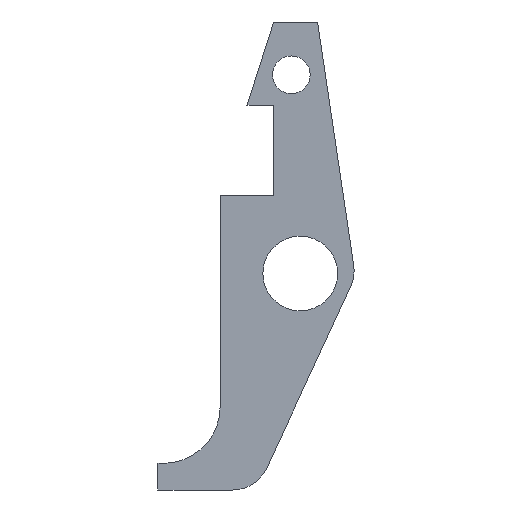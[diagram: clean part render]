
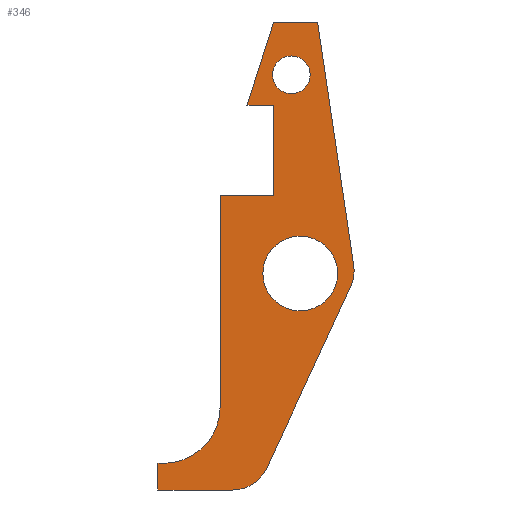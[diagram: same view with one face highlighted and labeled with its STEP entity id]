
A CAD part, front view. The second image highlights one B-rep face of the part: STEP entity #346.
In plain terms, the highlighted planar face has unit normal (0, -1, 0).
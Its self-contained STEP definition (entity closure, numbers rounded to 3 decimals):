
#17=FACE_BOUND('',#62,.T.);
#18=FACE_BOUND('',#63,.T.);
#19=CIRCLE('',#374,1.588);
#25=CIRCLE('',#383,3.175);
#26=CIRCLE('',#386,4.763);
#27=CIRCLE('',#387,3.175);
#28=CIRCLE('',#388,3.15);
#41=FACE_OUTER_BOUND('',#61,.T.);
#61=EDGE_LOOP('',(#270,#271,#272,#273,#274,#275,#276,#277,#278,#279,#280,
#281,#282,#283));
#62=EDGE_LOOP('',(#284));
#63=EDGE_LOOP('',(#285));
#76=LINE('',#503,#114);
#80=LINE('',#510,#118);
#82=LINE('',#519,#120);
#94=LINE('',#553,#132);
#96=LINE('',#557,#134);
#97=LINE('',#559,#135);
#98=LINE('',#561,#136);
#99=LINE('',#563,#137);
#100=LINE('',#567,#138);
#101=LINE('',#569,#139);
#102=LINE('',#571,#140);
#114=VECTOR('',#405,10.);
#118=VECTOR('',#411,10.);
#120=VECTOR('',#421,10.);
#132=VECTOR('',#449,10.);
#134=VECTOR('',#453,10.);
#135=VECTOR('',#454,10.);
#136=VECTOR('',#455,10.);
#137=VECTOR('',#456,10.);
#138=VECTOR('',#459,10.);
#139=VECTOR('',#460,10.);
#140=VECTOR('',#461,10.);
#152=VERTEX_POINT('',#500);
#153=VERTEX_POINT('',#502);
#155=VERTEX_POINT('',#508);
#156=VERTEX_POINT('',#512);
#158=VERTEX_POINT('',#518);
#171=VERTEX_POINT('',#548);
#172=VERTEX_POINT('',#552);
#173=VERTEX_POINT('',#556);
#174=VERTEX_POINT('',#558);
#175=VERTEX_POINT('',#560);
#176=VERTEX_POINT('',#562);
#177=VERTEX_POINT('',#564);
#178=VERTEX_POINT('',#566);
#179=VERTEX_POINT('',#568);
#180=VERTEX_POINT('',#570);
#181=VERTEX_POINT('',#573);
#184=EDGE_CURVE('',#153,#152,#76,.T.);
#188=EDGE_CURVE('',#152,#155,#80,.T.);
#189=EDGE_CURVE('',#156,#156,#19,.T.);
#192=EDGE_CURVE('',#158,#153,#82,.T.);
#207=EDGE_CURVE('',#158,#171,#25,.T.);
#209=EDGE_CURVE('',#172,#171,#94,.T.);
#211=EDGE_CURVE('',#155,#173,#96,.T.);
#212=EDGE_CURVE('',#173,#174,#97,.T.);
#213=EDGE_CURVE('',#174,#175,#98,.T.);
#214=EDGE_CURVE('',#175,#176,#99,.T.);
#215=EDGE_CURVE('',#177,#176,#26,.T.);
#216=EDGE_CURVE('',#177,#178,#100,.T.);
#217=EDGE_CURVE('',#178,#179,#101,.T.);
#218=EDGE_CURVE('',#179,#180,#102,.T.);
#219=EDGE_CURVE('',#172,#180,#27,.T.);
#220=EDGE_CURVE('',#181,#181,#28,.T.);
#270=ORIENTED_EDGE('',*,*,#188,.T.);
#271=ORIENTED_EDGE('',*,*,#211,.T.);
#272=ORIENTED_EDGE('',*,*,#212,.T.);
#273=ORIENTED_EDGE('',*,*,#213,.T.);
#274=ORIENTED_EDGE('',*,*,#214,.T.);
#275=ORIENTED_EDGE('',*,*,#215,.F.);
#276=ORIENTED_EDGE('',*,*,#216,.T.);
#277=ORIENTED_EDGE('',*,*,#217,.T.);
#278=ORIENTED_EDGE('',*,*,#218,.T.);
#279=ORIENTED_EDGE('',*,*,#219,.F.);
#280=ORIENTED_EDGE('',*,*,#209,.T.);
#281=ORIENTED_EDGE('',*,*,#207,.F.);
#282=ORIENTED_EDGE('',*,*,#192,.T.);
#283=ORIENTED_EDGE('',*,*,#184,.T.);
#284=ORIENTED_EDGE('',*,*,#189,.T.);
#285=ORIENTED_EDGE('',*,*,#220,.T.);
#331=PLANE('',#385);
#346=ADVANCED_FACE('',(#41,#17,#18),#331,.F.);
#374=AXIS2_PLACEMENT_3D('',#513,#414,#415);
#383=AXIS2_PLACEMENT_3D('',#549,#444,#445);
#385=AXIS2_PLACEMENT_3D('',#555,#451,#452);
#386=AXIS2_PLACEMENT_3D('',#565,#457,#458);
#387=AXIS2_PLACEMENT_3D('',#572,#462,#463);
#388=AXIS2_PLACEMENT_3D('',#574,#464,#465);
#405=DIRECTION('',(-1.,0.,0.));
#411=DIRECTION('',(-0.305,0.,-0.952));
#414=DIRECTION('center_axis',(0.,1.,0.));
#415=DIRECTION('ref_axis',(1.,0.,0.));
#421=DIRECTION('',(-0.147,0.,0.989));
#444=DIRECTION('center_axis',(0.,1.,0.));
#445=DIRECTION('ref_axis',(0.99,0.,-0.142));
#449=DIRECTION('',(0.42,0.,0.908));
#451=DIRECTION('center_axis',(0.,1.,0.));
#452=DIRECTION('ref_axis',(1.,0.,0.));
#453=DIRECTION('',(1.,0.,0.));
#454=DIRECTION('',(0.,0.,-1.));
#455=DIRECTION('',(-1.,0.,0.));
#456=DIRECTION('',(0.,0.,-1.));
#457=DIRECTION('center_axis',(0.,-1.,0.));
#458=DIRECTION('ref_axis',(0.707,0.,-0.707));
#459=DIRECTION('',(-1.,0.,0.));
#460=DIRECTION('',(0.,0.,-1.));
#461=DIRECTION('',(1.,0.,0.));
#462=DIRECTION('center_axis',(0.,1.,0.));
#463=DIRECTION('ref_axis',(0.539,0.,-0.843));
#464=DIRECTION('center_axis',(0.,1.,0.));
#465=DIRECTION('ref_axis',(1.,0.,0.));
#500=CARTESIAN_POINT('',(-7.746,-0.794,-58.733));
#502=CARTESIAN_POINT('',(-4.034,-0.794,-58.733));
#503=CARTESIAN_POINT('',(-6.604,-0.794,-58.733));
#508=CARTESIAN_POINT('',(-9.988,-0.794,-65.733));
#510=CARTESIAN_POINT('',(-10.075,-0.794,-66.003));
#512=CARTESIAN_POINT('',(-7.838,-0.794,-63.183));
#513=CARTESIAN_POINT('Origin',(-6.25,-0.794,-63.183));
#518=CARTESIAN_POINT('',(-0.989,-0.794,-79.245));
#519=CARTESIAN_POINT('',(-0.85,-0.794,-80.183));
#548=CARTESIAN_POINT('',(-1.248,-0.794,-81.044));
#549=CARTESIAN_POINT('Origin',(-4.13,-0.794,-79.711));
#552=CARTESIAN_POINT('',(-8.323,-0.794,-96.341));
#553=CARTESIAN_POINT('',(-9.176,-0.794,-98.183));
#555=CARTESIAN_POINT('Origin',(-9.175,-0.794,-74.308));
#556=CARTESIAN_POINT('',(-7.75,-0.794,-65.733));
#557=CARTESIAN_POINT('',(-7.75,-0.794,-65.733));
#558=CARTESIAN_POINT('',(-7.75,-0.794,-73.383));
#559=CARTESIAN_POINT('',(-7.75,-0.794,-73.383));
#560=CARTESIAN_POINT('',(-12.25,-0.794,-73.383));
#561=CARTESIAN_POINT('',(-12.25,-0.794,-73.383));
#562=CARTESIAN_POINT('',(-12.25,-0.794,-91.171));
#563=CARTESIAN_POINT('',(-12.25,-0.794,-80.183));
#564=CARTESIAN_POINT('',(-17.013,-0.794,-95.933));
#565=CARTESIAN_POINT('Origin',(-17.013,-0.794,-91.171));
#566=CARTESIAN_POINT('',(-17.5,-0.794,-95.933));
#567=CARTESIAN_POINT('',(-12.25,-0.794,-95.933));
#568=CARTESIAN_POINT('',(-17.5,-0.794,-98.183));
#569=CARTESIAN_POINT('',(-17.5,-0.794,-95.933));
#570=CARTESIAN_POINT('',(-11.205,-0.794,-98.183));
#571=CARTESIAN_POINT('',(-17.5,-0.794,-98.183));
#572=CARTESIAN_POINT('Origin',(-11.205,-0.794,-95.008));
#573=CARTESIAN_POINT('',(-8.65,-0.794,-79.933));
#574=CARTESIAN_POINT('Origin',(-5.5,-0.794,-79.933));
